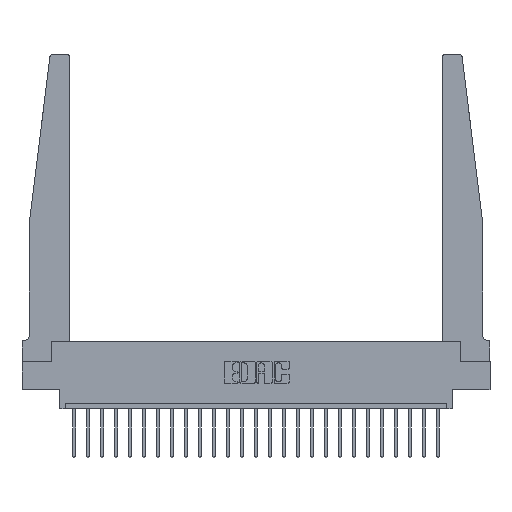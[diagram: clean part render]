
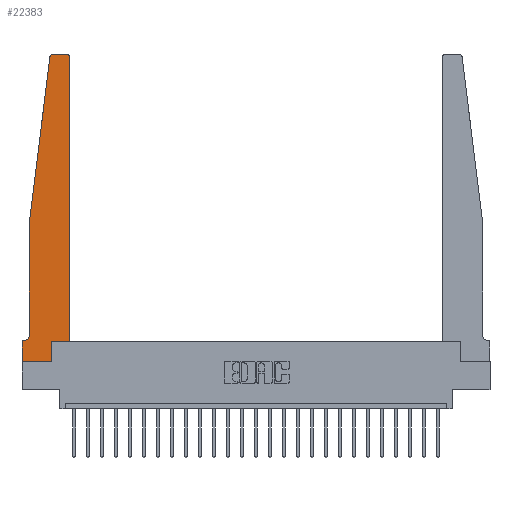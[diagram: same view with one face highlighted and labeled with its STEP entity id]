
A CAD part, top view. The second image highlights one B-rep face of the part: STEP entity #22383.
In plain terms, the highlighted planar face has unit normal (0, 0, 1).
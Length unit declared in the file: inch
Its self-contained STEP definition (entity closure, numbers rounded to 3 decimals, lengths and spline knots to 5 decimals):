
#27 = EDGE_CURVE ( 'NONE', #871, #6892, #18363, .T. ) ;
#56 = DIRECTION ( 'NONE',  ( 1., 0., 0. ) ) ;
#129 = VECTOR ( 'NONE', #8997, 39.37008 ) ;
#871 = VERTEX_POINT ( 'NONE', #2086 ) ;
#974 = CARTESIAN_POINT ( 'NONE',  ( 0.065, 0.1875, 0.37 ) ) ;
#1535 = CARTESIAN_POINT ( 'NONE',  ( 0.2605, 0.18, 0.37 ) ) ;
#1550 = LINE ( 'NONE', #18385, #12195 ) ;
#1649 = VERTEX_POINT ( 'NONE', #3060 ) ;
#1663 = EDGE_CURVE ( 'NONE', #5536, #871, #1811, .T. ) ;
#1664 = CARTESIAN_POINT ( 'NONE',  ( 0., 0.1875, 0.37 ) ) ;
#1811 = LINE ( 'NONE', #4962, #8119 ) ;
#1868 = CARTESIAN_POINT ( 'NONE',  ( 0., 0., 0.37 ) ) ;
#2086 = CARTESIAN_POINT ( 'NONE',  ( 0., 0., 0.37 ) ) ;
#2205 = LINE ( 'NONE', #14567, #5615 ) ;
#2268 = CARTESIAN_POINT ( 'NONE',  ( 0., 0.1875, 0.37 ) ) ;
#2442 = ORIENTED_EDGE ( 'NONE', *, *, #16191, .T. ) ;
#2475 = AXIS2_PLACEMENT_3D ( 'NONE', #2268, #7696, #22275 ) ;
#2588 = VERTEX_POINT ( 'NONE', #4896 ) ;
#2673 = LINE ( 'NONE', #974, #4070 ) ;
#3060 = CARTESIAN_POINT ( 'NONE',  ( 0.27653, 2.75, 0.37 ) ) ;
#3721 = ORIENTED_EDGE ( 'NONE', *, *, #9901, .T. ) ;
#3978 = DIRECTION ( 'NONE',  ( 0., 1., 0. ) ) ;
#4070 = VECTOR ( 'NONE', #23302, 39.37008 ) ;
#4602 = VECTOR ( 'NONE', #56, 39.37008 ) ;
#4794 = VECTOR ( 'NONE', #20901, 39.37008 ) ;
#4896 = CARTESIAN_POINT ( 'NONE',  ( 0.065, 1.25, 0.37 ) ) ;
#4962 = CARTESIAN_POINT ( 'NONE',  ( 0., 0., 0.37 ) ) ;
#5179 = DIRECTION ( 'NONE',  ( -0.122, -0.992, 0. ) ) ;
#5206 = FACE_OUTER_BOUND ( 'NONE', #8932, .T. ) ;
#5536 = VERTEX_POINT ( 'NONE', #1664 ) ;
#5588 = ORIENTED_EDGE ( 'NONE', *, *, #7275, .T. ) ;
#5615 = VECTOR ( 'NONE', #19926, 39.37008 ) ;
#5636 = VECTOR ( 'NONE', #8628, 39.37008 ) ;
#5823 = CARTESIAN_POINT ( 'NONE',  ( 0.425, 0.18, 0.37 ) ) ;
#6030 = CIRCLE ( 'NONE', #21174, 0.05 ) ;
#6558 = ORIENTED_EDGE ( 'NONE', *, *, #20828, .T. ) ;
#6768 = DIRECTION ( 'NONE',  ( -1., 0., 0. ) ) ;
#6892 = VERTEX_POINT ( 'NONE', #14993 ) ;
#6989 = CARTESIAN_POINT ( 'NONE',  ( 0.25, 2.75, 0.37 ) ) ;
#7275 = EDGE_CURVE ( 'NONE', #15237, #1649, #9110, .T. ) ;
#7696 = DIRECTION ( 'NONE',  ( 0., 0., 1. ) ) ;
#7805 = CARTESIAN_POINT ( 'NONE',  ( 0.425, 0.18, 0.37 ) ) ;
#7964 = AXIS2_PLACEMENT_3D ( 'NONE', #8841, #10769, #23560 ) ;
#8119 = VECTOR ( 'NONE', #12127, 39.37008 ) ;
#8587 = VERTEX_POINT ( 'NONE', #13606 ) ;
#8628 = DIRECTION ( 'NONE',  ( -1., 0., 0. ) ) ;
#8841 = CARTESIAN_POINT ( 'NONE',  ( 0.395, 2.72, 0.37 ) ) ;
#8932 = EDGE_LOOP ( 'NONE', ( #5588, #2442, #10132, #16864, #21239, #16474, #18583, #21846, #6558, #22063, #17832, #3721 ) ) ;
#8997 = DIRECTION ( 'NONE',  ( 0., 1., 0. ) ) ;
#9110 = LINE ( 'NONE', #6989, #5636 ) ;
#9130 = EDGE_CURVE ( 'NONE', #16559, #2588, #11881, .T. ) ;
#9547 = DIRECTION ( 'NONE',  ( 1., 0., 0. ) ) ;
#9612 = LINE ( 'NONE', #1535, #129 ) ;
#9901 = EDGE_CURVE ( 'NONE', #17191, #15237, #18965, .T. ) ;
#10132 = ORIENTED_EDGE ( 'NONE', *, *, #9130, .T. ) ;
#10516 = LINE ( 'NONE', #7805, #4794 ) ;
#10769 = DIRECTION ( 'NONE',  ( 0., 0., 1. ) ) ;
#10881 = CARTESIAN_POINT ( 'NONE',  ( 0.065, 1.25, 0.37 ) ) ;
#10893 = CARTESIAN_POINT ( 'NONE',  ( 0.425, 2.72, 0.37 ) ) ;
#11406 = PLANE ( 'NONE',  #2475 ) ;
#11780 = VERTEX_POINT ( 'NONE', #22721 ) ;
#11881 = LINE ( 'NONE', #10881, #13884 ) ;
#12088 = EDGE_CURVE ( 'NONE', #8587, #5536, #2673, .T. ) ;
#12127 = DIRECTION ( 'NONE',  ( 0., -1., 0. ) ) ;
#12195 = VECTOR ( 'NONE', #3978, 39.37008 ) ;
#13395 = DIRECTION ( 'NONE',  ( 0., 0., 1. ) ) ;
#13606 = CARTESIAN_POINT ( 'NONE',  ( 0.015, 0.1875, 0.37 ) ) ;
#13884 = VECTOR ( 'NONE', #5179, 39.37008 ) ;
#13936 = AXIS2_PLACEMENT_3D ( 'NONE', #20455, #13395, #9547 ) ;
#14567 = CARTESIAN_POINT ( 'NONE',  ( 0.065, 1.25, 0.37 ) ) ;
#14993 = CARTESIAN_POINT ( 'NONE',  ( 0.2605, 0., 0.37 ) ) ;
#15237 = VERTEX_POINT ( 'NONE', #17637 ) ;
#16191 = EDGE_CURVE ( 'NONE', #1649, #16559, #17902, .T. ) ;
#16474 = ORIENTED_EDGE ( 'NONE', *, *, #12088, .T. ) ;
#16559 = VERTEX_POINT ( 'NONE', #18642 ) ;
#16864 = ORIENTED_EDGE ( 'NONE', *, *, #19391, .T. ) ;
#17191 = VERTEX_POINT ( 'NONE', #10893 ) ;
#17287 = VERTEX_POINT ( 'NONE', #20608 ) ;
#17637 = CARTESIAN_POINT ( 'NONE',  ( 0.395, 2.75, 0.37 ) ) ;
#17772 = DIRECTION ( 'NONE',  ( 0., 0., -1. ) ) ;
#17832 = ORIENTED_EDGE ( 'NONE', *, *, #20549, .T. ) ;
#17854 = CARTESIAN_POINT ( 'NONE',  ( 0.015, 0.2375, 0.37 ) ) ;
#17902 = CIRCLE ( 'NONE', #13936, 0.03 ) ;
#18363 = LINE ( 'NONE', #1868, #4602 ) ;
#18385 = CARTESIAN_POINT ( 'NONE',  ( 0.425, 0.18, 0.37 ) ) ;
#18583 = ORIENTED_EDGE ( 'NONE', *, *, #1663, .T. ) ;
#18642 = CARTESIAN_POINT ( 'NONE',  ( 0.24675, 2.72367, 0.37 ) ) ;
#18965 = CIRCLE ( 'NONE', #7964, 0.03 ) ;
#19092 = EDGE_CURVE ( 'NONE', #11780, #20230, #10516, .T. ) ;
#19391 = EDGE_CURVE ( 'NONE', #2588, #17287, #2205, .T. ) ;
#19926 = DIRECTION ( 'NONE',  ( 0., -1., 0. ) ) ;
#20230 = VERTEX_POINT ( 'NONE', #5823 ) ;
#20455 = CARTESIAN_POINT ( 'NONE',  ( 0.27653, 2.72, 0.37 ) ) ;
#20549 = EDGE_CURVE ( 'NONE', #20230, #17191, #1550, .T. ) ;
#20608 = CARTESIAN_POINT ( 'NONE',  ( 0.065, 0.2375, 0.37 ) ) ;
#20828 = EDGE_CURVE ( 'NONE', #6892, #11780, #9612, .T. ) ;
#20901 = DIRECTION ( 'NONE',  ( 1., 0., 0. ) ) ;
#21174 = AXIS2_PLACEMENT_3D ( 'NONE', #17854, #17772, #6768 ) ;
#21239 = ORIENTED_EDGE ( 'NONE', *, *, #22579, .T. ) ;
#21846 = ORIENTED_EDGE ( 'NONE', *, *, #27, .T. ) ;
#22063 = ORIENTED_EDGE ( 'NONE', *, *, #19092, .T. ) ;
#22275 = DIRECTION ( 'NONE',  ( 1., 0., 0. ) ) ;
#22383 = ADVANCED_FACE ( 'NONE', ( #5206 ), #11406, .T. ) ;
#22579 = EDGE_CURVE ( 'NONE', #17287, #8587, #6030, .T. ) ;
#22721 = CARTESIAN_POINT ( 'NONE',  ( 0.2605, 0.18, 0.37 ) ) ;
#23302 = DIRECTION ( 'NONE',  ( -1., 0., 0. ) ) ;
#23560 = DIRECTION ( 'NONE',  ( 1., 0., 0. ) ) ;
